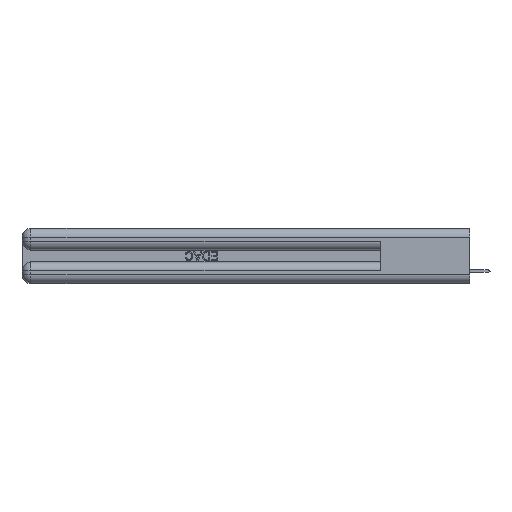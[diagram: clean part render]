
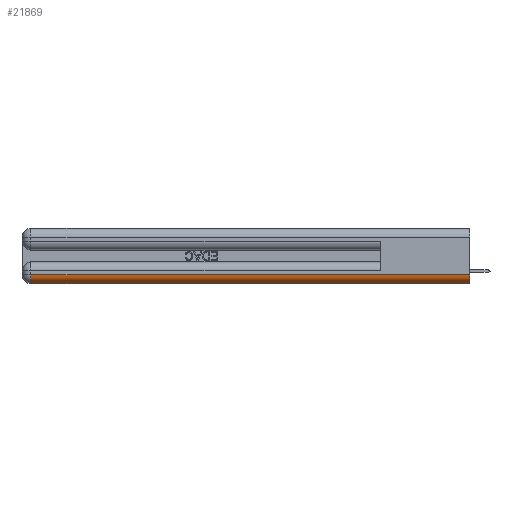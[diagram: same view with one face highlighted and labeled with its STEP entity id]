
A CAD part, left-side view. The second image highlights one B-rep face of the part: STEP entity #21869.
In plain terms, the highlighted cylindrical face has radius 1.524 mm (diameter 3.048 mm), a partial arc.
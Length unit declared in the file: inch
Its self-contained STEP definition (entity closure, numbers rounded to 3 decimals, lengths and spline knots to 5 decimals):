
#1248 = DIRECTION ( 'NONE',  ( 0., -1., 0. ) ) ;
#1694 = EDGE_LOOP ( 'NONE', ( #5935, #45988, #7668, #4147 ) ) ;
#2281 = CARTESIAN_POINT ( 'NONE',  ( 0.06, 3., 0. ) ) ;
#4147 = ORIENTED_EDGE ( 'NONE', *, *, #19980, .F. ) ;
#5119 = DIRECTION ( 'NONE',  ( 0., 1., 0. ) ) ;
#5935 = ORIENTED_EDGE ( 'NONE', *, *, #44794, .F. ) ;
#7668 = ORIENTED_EDGE ( 'NONE', *, *, #25313, .F. ) ;
#8565 = VERTEX_POINT ( 'NONE', #9311 ) ;
#8614 = CARTESIAN_POINT ( 'NONE',  ( 0.06, 0., 0.06 ) ) ;
#9311 = CARTESIAN_POINT ( 'NONE',  ( 0., 0., 0.06 ) ) ;
#9499 = VECTOR ( 'NONE', #19849, 39.37008 ) ;
#9769 = VERTEX_POINT ( 'NONE', #38220 ) ;
#11572 = AXIS2_PLACEMENT_3D ( 'NONE', #19546, #12348, #23011 ) ;
#11766 = VERTEX_POINT ( 'NONE', #37061 ) ;
#12348 = DIRECTION ( 'NONE',  ( 0., 1., 0. ) ) ;
#13265 = CIRCLE ( 'NONE', #42249, 0.06 ) ;
#13952 = EDGE_CURVE ( 'NONE', #44482, #8565, #23545, .T. ) ;
#19546 = CARTESIAN_POINT ( 'NONE',  ( 0.06, 2.94, 0.06 ) ) ;
#19849 = DIRECTION ( 'NONE',  ( 0., -1., 0. ) ) ;
#19980 = EDGE_CURVE ( 'NONE', #9769, #11766, #33294, .T. ) ;
#20994 = VECTOR ( 'NONE', #23463, 39.37008 ) ;
#21869 = ADVANCED_FACE ( 'NONE', ( #33309 ), #37045, .T. ) ;
#23011 = DIRECTION ( 'NONE',  ( 0., 0., 1. ) ) ;
#23463 = DIRECTION ( 'NONE',  ( 0., 1., 0. ) ) ;
#23545 = LINE ( 'NONE', #34296, #9499 ) ;
#25313 = EDGE_CURVE ( 'NONE', #11766, #44482, #31606, .T. ) ;
#26197 = DIRECTION ( 'NONE',  ( 0., 0., 1. ) ) ;
#27840 = CARTESIAN_POINT ( 'NONE',  ( 0., 2.94, 0.06 ) ) ;
#30358 = CARTESIAN_POINT ( 'NONE',  ( 0.06, 0., 0.06 ) ) ;
#31606 = CIRCLE ( 'NONE', #11572, 0.06 ) ;
#33294 = LINE ( 'NONE', #2281, #20994 ) ;
#33309 = FACE_OUTER_BOUND ( 'NONE', #1694, .T. ) ;
#34296 = CARTESIAN_POINT ( 'NONE',  ( 0., 0., 0.06 ) ) ;
#37045 = CYLINDRICAL_SURFACE ( 'NONE', #37417, 0.06 ) ;
#37061 = CARTESIAN_POINT ( 'NONE',  ( 0.06, 2.94, 0. ) ) ;
#37417 = AXIS2_PLACEMENT_3D ( 'NONE', #8614, #5119, #44519 ) ;
#38220 = CARTESIAN_POINT ( 'NONE',  ( 0.06, 0., 0. ) ) ;
#42249 = AXIS2_PLACEMENT_3D ( 'NONE', #30358, #1248, #26197 ) ;
#44482 = VERTEX_POINT ( 'NONE', #27840 ) ;
#44519 = DIRECTION ( 'NONE',  ( 0., 0., 1. ) ) ;
#44794 = EDGE_CURVE ( 'NONE', #8565, #9769, #13265, .T. ) ;
#45988 = ORIENTED_EDGE ( 'NONE', *, *, #13952, .F. ) ;
